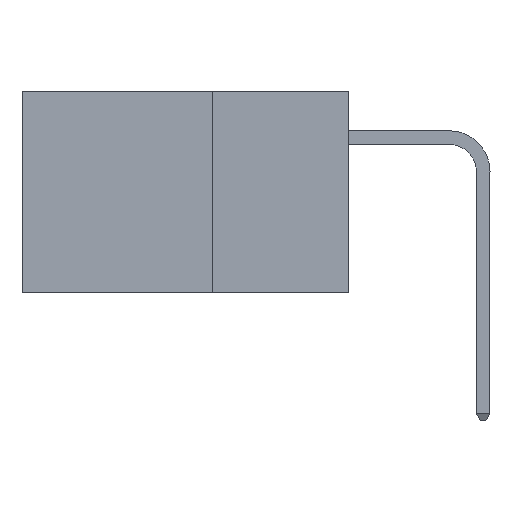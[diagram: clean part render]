
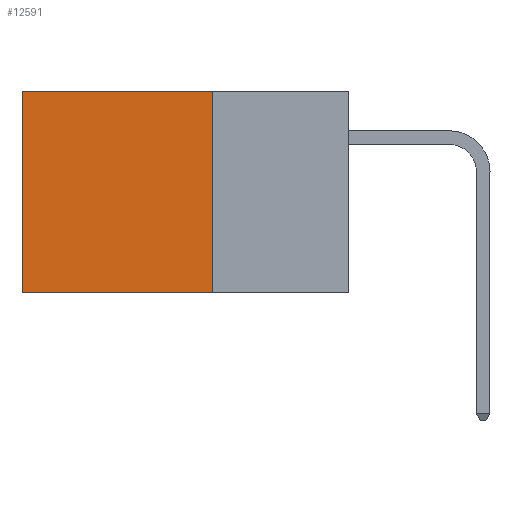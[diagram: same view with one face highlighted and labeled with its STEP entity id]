
A CAD part, left-side view. The second image highlights one B-rep face of the part: STEP entity #12591.
In plain terms, the highlighted planar face has unit normal (-1, 0, 0).
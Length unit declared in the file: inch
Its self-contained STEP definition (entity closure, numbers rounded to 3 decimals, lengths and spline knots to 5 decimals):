
#1112 = DIRECTION ( 'NONE',  ( 0., 0., -1. ) ) ;
#1179 = VECTOR ( 'NONE', #1112, 39.37008 ) ;
#1773 = ORIENTED_EDGE ( 'NONE', *, *, #9873, .T. ) ;
#3483 = VERTEX_POINT ( 'NONE', #4104 ) ;
#3868 = EDGE_CURVE ( 'NONE', #18228, #3483, #12142, .T. ) ;
#4104 = CARTESIAN_POINT ( 'NONE',  ( 0.2875, 0.25, -0.37 ) ) ;
#4241 = VERTEX_POINT ( 'NONE', #11088 ) ;
#6249 = DIRECTION ( 'NONE',  ( 0., 0., -1. ) ) ;
#6660 = VERTEX_POINT ( 'NONE', #21978 ) ;
#8088 = VECTOR ( 'NONE', #11448, 39.37008 ) ;
#8557 = CARTESIAN_POINT ( 'NONE',  ( 0.2875, 0.25, 0. ) ) ;
#8972 = ORIENTED_EDGE ( 'NONE', *, *, #24282, .F. ) ;
#9728 = DIRECTION ( 'NONE',  ( 0., 1., 0. ) ) ;
#9873 = EDGE_CURVE ( 'NONE', #4241, #6660, #21647, .T. ) ;
#10388 = CARTESIAN_POINT ( 'NONE',  ( 0.2875, 0.25, 0. ) ) ;
#10691 = EDGE_CURVE ( 'NONE', #18228, #4241, #23948, .T. ) ;
#10712 = CARTESIAN_POINT ( 'NONE',  ( 0.2875, 0.6, 0. ) ) ;
#11088 = CARTESIAN_POINT ( 'NONE',  ( 0.2875, 0.6, 0. ) ) ;
#11448 = DIRECTION ( 'NONE',  ( 0., 1., 0. ) ) ;
#12142 = LINE ( 'NONE', #13866, #16046 ) ;
#12416 = DIRECTION ( 'NONE',  ( 0., 0., -1. ) ) ;
#12591 = ADVANCED_FACE ( 'NONE', ( #19168 ), #14241, .F. ) ;
#13807 = VECTOR ( 'NONE', #9728, 39.37008 ) ;
#13866 = CARTESIAN_POINT ( 'NONE',  ( 0.2875, 0.25, 0. ) ) ;
#14241 = PLANE ( 'NONE',  #16617 ) ;
#15106 = EDGE_LOOP ( 'NONE', ( #1773, #8972, #20797, #23588 ) ) ;
#16046 = VECTOR ( 'NONE', #6249, 39.37008 ) ;
#16617 = AXIS2_PLACEMENT_3D ( 'NONE', #8557, #23866, #12416 ) ;
#18228 = VERTEX_POINT ( 'NONE', #10388 ) ;
#19168 = FACE_OUTER_BOUND ( 'NONE', #15106, .T. ) ;
#19361 = CARTESIAN_POINT ( 'NONE',  ( 0.2875, 0.25, -0.37 ) ) ;
#20797 = ORIENTED_EDGE ( 'NONE', *, *, #3868, .F. ) ;
#21009 = CARTESIAN_POINT ( 'NONE',  ( 0.2875, 0.25, 0. ) ) ;
#21647 = LINE ( 'NONE', #10712, #1179 ) ;
#21978 = CARTESIAN_POINT ( 'NONE',  ( 0.2875, 0.6, -0.37 ) ) ;
#23588 = ORIENTED_EDGE ( 'NONE', *, *, #10691, .T. ) ;
#23866 = DIRECTION ( 'NONE',  ( 1., 0., 0. ) ) ;
#23948 = LINE ( 'NONE', #21009, #8088 ) ;
#23986 = LINE ( 'NONE', #19361, #13807 ) ;
#24282 = EDGE_CURVE ( 'NONE', #3483, #6660, #23986, .T. ) ;
